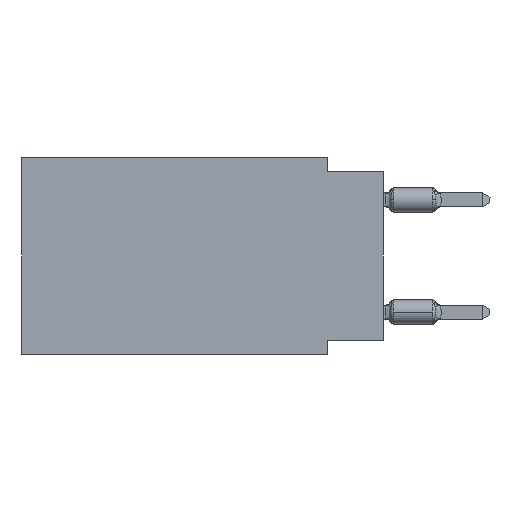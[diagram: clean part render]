
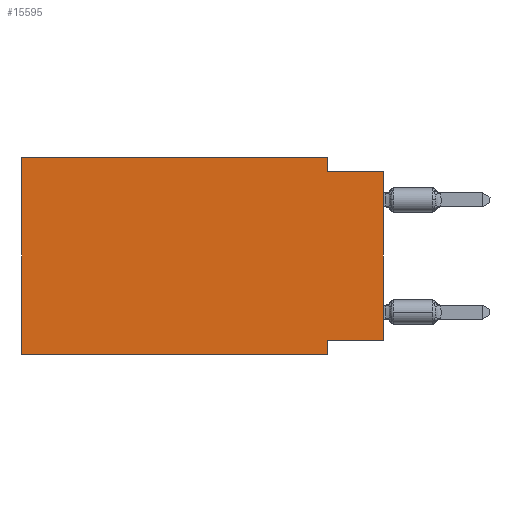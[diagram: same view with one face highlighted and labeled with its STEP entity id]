
A CAD part, left-side view. The second image highlights one B-rep face of the part: STEP entity #15595.
In plain terms, the highlighted planar face has unit normal (-1, 0, 0).
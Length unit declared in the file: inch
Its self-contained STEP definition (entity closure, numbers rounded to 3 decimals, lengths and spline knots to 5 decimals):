
#579 = VECTOR ( 'NONE', #1890, 39.37008 ) ;
#835 = DIRECTION ( 'NONE',  ( 1., 0., 0. ) ) ;
#918 = CARTESIAN_POINT ( 'NONE',  ( 0., 0.645, 0. ) ) ;
#1001 = VECTOR ( 'NONE', #5127, 39.37008 ) ;
#1011 = CARTESIAN_POINT ( 'NONE',  ( 0., 0.1, 0. ) ) ;
#1060 = FACE_OUTER_BOUND ( 'NONE', #2287, .T. ) ;
#1079 = CARTESIAN_POINT ( 'NONE',  ( 0., 0., 0. ) ) ;
#1145 = LINE ( 'NONE', #15982, #2393 ) ;
#1307 = EDGE_CURVE ( 'NONE', #15523, #19612, #2089, .T. ) ;
#1815 = ORIENTED_EDGE ( 'NONE', *, *, #17214, .F. ) ;
#1890 = DIRECTION ( 'NONE',  ( 0., -1., 0. ) ) ;
#2036 = ORIENTED_EDGE ( 'NONE', *, *, #1307, .T. ) ;
#2089 = LINE ( 'NONE', #3539, #579 ) ;
#2287 = EDGE_LOOP ( 'NONE', ( #4720, #21340, #7319, #1815, #5657, #2036, #8870, #10930 ) ) ;
#2292 = CARTESIAN_POINT ( 'NONE',  ( 0., 0., -0.325 ) ) ;
#2393 = VECTOR ( 'NONE', #21185, 39.37008 ) ;
#2673 = CARTESIAN_POINT ( 'NONE',  ( 0., 0.645, -0.35 ) ) ;
#2991 = DIRECTION ( 'NONE',  ( 0., 0., 1. ) ) ;
#3084 = EDGE_CURVE ( 'NONE', #21006, #5673, #21009, .T. ) ;
#3539 = CARTESIAN_POINT ( 'NONE',  ( 0., 0.645, -0.35 ) ) ;
#4525 = VECTOR ( 'NONE', #2991, 39.37008 ) ;
#4637 = CARTESIAN_POINT ( 'NONE',  ( 0., 0.1, -0.325 ) ) ;
#4668 = DIRECTION ( 'NONE',  ( 0., 0., -1. ) ) ;
#4720 = ORIENTED_EDGE ( 'NONE', *, *, #3084, .T. ) ;
#4812 = AXIS2_PLACEMENT_3D ( 'NONE', #11106, #835, #20763 ) ;
#5127 = DIRECTION ( 'NONE',  ( 0., 0., -1. ) ) ;
#5657 = ORIENTED_EDGE ( 'NONE', *, *, #17082, .F. ) ;
#5673 = VERTEX_POINT ( 'NONE', #7710 ) ;
#5762 = CARTESIAN_POINT ( 'NONE',  ( 0., 0.645, 0. ) ) ;
#5994 = CARTESIAN_POINT ( 'NONE',  ( 0., 0.1, -0.35 ) ) ;
#6689 = CARTESIAN_POINT ( 'NONE',  ( 0., 0.1, 0. ) ) ;
#7319 = ORIENTED_EDGE ( 'NONE', *, *, #9166, .F. ) ;
#7710 = CARTESIAN_POINT ( 'NONE',  ( 0., 0., -0.025 ) ) ;
#8722 = VERTEX_POINT ( 'NONE', #1011 ) ;
#8870 = ORIENTED_EDGE ( 'NONE', *, *, #15497, .F. ) ;
#9106 = CARTESIAN_POINT ( 'NONE',  ( 0., 0.1, -0.35 ) ) ;
#9166 = EDGE_CURVE ( 'NONE', #8722, #15480, #18350, .T. ) ;
#9176 = DIRECTION ( 'NONE',  ( 0., 0., 1. ) ) ;
#10930 = ORIENTED_EDGE ( 'NONE', *, *, #19658, .F. ) ;
#11106 = CARTESIAN_POINT ( 'NONE',  ( 0., 0.645, 0. ) ) ;
#11842 = VECTOR ( 'NONE', #9176, 39.37008 ) ;
#12409 = DIRECTION ( 'NONE',  ( 0., -1., 0. ) ) ;
#12634 = CARTESIAN_POINT ( 'NONE',  ( 0., 0.1, -0.025 ) ) ;
#13339 = CARTESIAN_POINT ( 'NONE',  ( 0., 0., -0.325 ) ) ;
#14566 = LINE ( 'NONE', #19483, #4525 ) ;
#14904 = EDGE_CURVE ( 'NONE', #15480, #5673, #1145, .T. ) ;
#15480 = VERTEX_POINT ( 'NONE', #12634 ) ;
#15497 = EDGE_CURVE ( 'NONE', #18151, #19612, #20887, .T. ) ;
#15523 = VERTEX_POINT ( 'NONE', #2673 ) ;
#15595 = ADVANCED_FACE ( 'NONE', ( #1060 ), #20992, .F. ) ;
#15635 = DIRECTION ( 'NONE',  ( 0., 1., 0. ) ) ;
#15982 = CARTESIAN_POINT ( 'NONE',  ( 0., 0., -0.025 ) ) ;
#16682 = VECTOR ( 'NONE', #4668, 39.37008 ) ;
#17082 = EDGE_CURVE ( 'NONE', #15523, #20548, #14566, .T. ) ;
#17214 = EDGE_CURVE ( 'NONE', #20548, #8722, #18755, .T. ) ;
#17273 = LINE ( 'NONE', #2292, #17358 ) ;
#17358 = VECTOR ( 'NONE', #15635, 39.37008 ) ;
#18151 = VERTEX_POINT ( 'NONE', #4637 ) ;
#18350 = LINE ( 'NONE', #6689, #1001 ) ;
#18755 = LINE ( 'NONE', #5762, #20842 ) ;
#19483 = CARTESIAN_POINT ( 'NONE',  ( 0., 0.645, 0. ) ) ;
#19612 = VERTEX_POINT ( 'NONE', #9106 ) ;
#19658 = EDGE_CURVE ( 'NONE', #21006, #18151, #17273, .T. ) ;
#20548 = VERTEX_POINT ( 'NONE', #918 ) ;
#20763 = DIRECTION ( 'NONE',  ( 0., 0., -1. ) ) ;
#20842 = VECTOR ( 'NONE', #12409, 39.37008 ) ;
#20887 = LINE ( 'NONE', #5994, #16682 ) ;
#20992 = PLANE ( 'NONE',  #4812 ) ;
#21006 = VERTEX_POINT ( 'NONE', #13339 ) ;
#21009 = LINE ( 'NONE', #1079, #11842 ) ;
#21185 = DIRECTION ( 'NONE',  ( 0., -1., 0. ) ) ;
#21340 = ORIENTED_EDGE ( 'NONE', *, *, #14904, .F. ) ;
